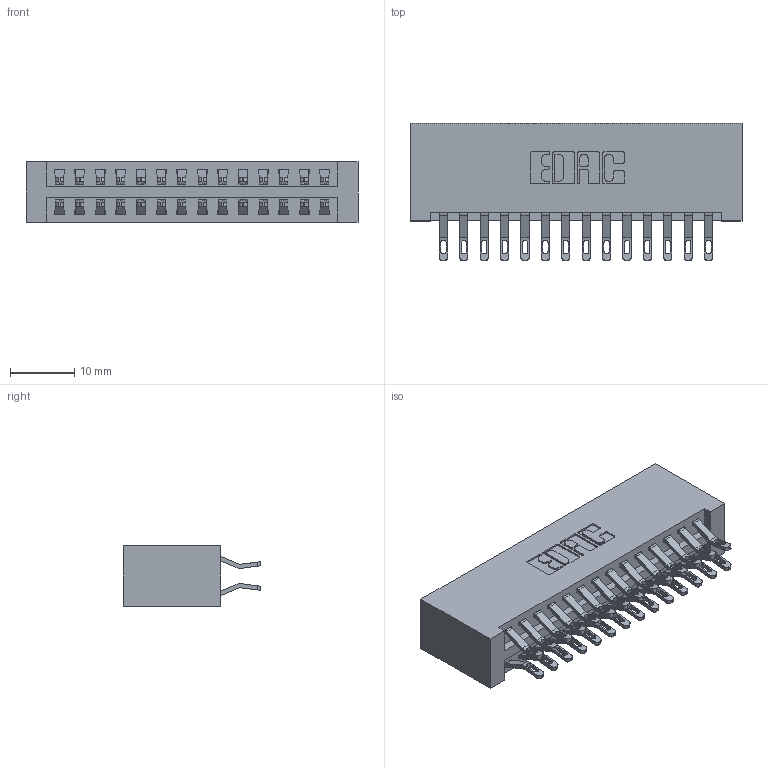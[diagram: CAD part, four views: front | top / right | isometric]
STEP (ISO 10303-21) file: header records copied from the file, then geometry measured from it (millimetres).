
FILE_DESCRIPTION (( 'STEP AP203' ), '1' );
FILE_NAME ('396-028-555-201.STEP', '2019-10-30T05:21:43', ( '' ), ( '' ), 'SwSTEP 2.0', 'SolidWorks 2016', '' );
FILE_SCHEMA (( 'CONFIG_CONTROL_DESIGN' ));
Length unit declared in the file: inch
Products named in the file (3): 396-028-555-201; 345-292-001_555 Tail; 346 Part_No Mounting Lugs
Assembly tree (29 placements, depth 2):
  396-028-555-201
    346 Part_No Mounting Lugs
    345-292-001_555 Tail  x28
Bounding box: 51.69 x 21.46 x 9.4 mm (x, y, z)
Volume: 5477.3 mm3; surface area: 7541.6 mm2
Topology: 29 solids, 29 shells, 1738 faces, 5429 edges, 3618 vertices
Faces by surface type: plane 996, cylinder 742
Entity records: 12955 total; most frequent: CARTESIAN_POINT 2206, ORIENTED_EDGE 2110, DIRECTION 1959, EDGE_CURVE 1055, LINE 855, VECTOR 855, VERTEX_POINT 702, AXIS2_PLACEMENT_3D 552
